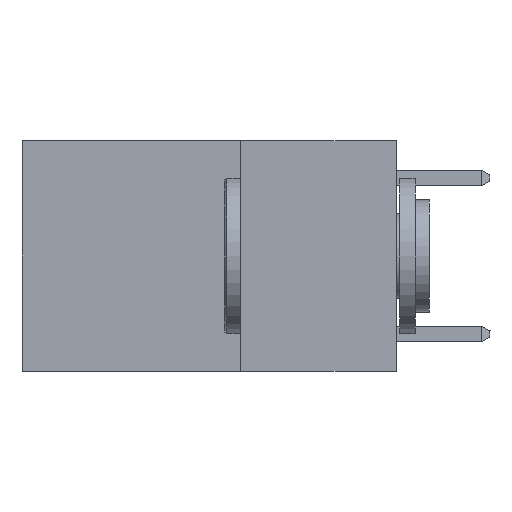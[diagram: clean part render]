
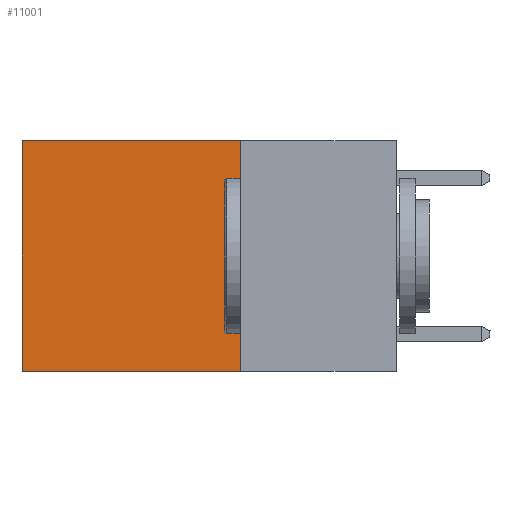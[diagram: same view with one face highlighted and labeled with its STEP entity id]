
A CAD part, left-side view. The second image highlights one B-rep face of the part: STEP entity #11001.
In plain terms, the highlighted planar face has unit normal (-1, 0, 0).
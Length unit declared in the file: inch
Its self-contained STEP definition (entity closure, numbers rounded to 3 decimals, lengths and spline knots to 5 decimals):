
#220 = PLANE ( 'NONE',  #23962 ) ;
#260 = CARTESIAN_POINT ( 'NONE',  ( 0.2625, 0.25, 0. ) ) ;
#681 = CARTESIAN_POINT ( 'NONE',  ( 0.2625, 0.25, -0.37 ) ) ;
#1607 = DIRECTION ( 'NONE',  ( 0., 0., -1. ) ) ;
#2259 = DIRECTION ( 'NONE',  ( 0., 1., 0. ) ) ;
#2545 = DIRECTION ( 'NONE',  ( 1., 0., 0. ) ) ;
#2746 = FACE_OUTER_BOUND ( 'NONE', #20581, .T. ) ;
#4446 = VECTOR ( 'NONE', #2259, 39.37008 ) ;
#4659 = ORIENTED_EDGE ( 'NONE', *, *, #26572, .T. ) ;
#5555 = ORIENTED_EDGE ( 'NONE', *, *, #27954, .F. ) ;
#5830 = LINE ( 'NONE', #10187, #11210 ) ;
#5943 = VERTEX_POINT ( 'NONE', #260 ) ;
#7524 = VERTEX_POINT ( 'NONE', #7734 ) ;
#7734 = CARTESIAN_POINT ( 'NONE',  ( 0.2625, 0.25, -0.37 ) ) ;
#8645 = VECTOR ( 'NONE', #18981, 39.37008 ) ;
#9068 = CARTESIAN_POINT ( 'NONE',  ( 0.2625, 0.25, 0. ) ) ;
#10187 = CARTESIAN_POINT ( 'NONE',  ( 0.2625, 0.25, 0. ) ) ;
#10566 = LINE ( 'NONE', #9068, #4446 ) ;
#11001 = ADVANCED_FACE ( 'NONE', ( #2746 ), #220, .F. ) ;
#11210 = VECTOR ( 'NONE', #16945, 39.37008 ) ;
#12831 = EDGE_CURVE ( 'NONE', #5943, #27323, #10566, .T. ) ;
#16250 = CARTESIAN_POINT ( 'NONE',  ( 0.2625, 0.25, 0. ) ) ;
#16945 = DIRECTION ( 'NONE',  ( 0., 0., -1. ) ) ;
#18523 = DIRECTION ( 'NONE',  ( 0., 0., -1. ) ) ;
#18981 = DIRECTION ( 'NONE',  ( 0., 1., 0. ) ) ;
#19715 = ORIENTED_EDGE ( 'NONE', *, *, #23733, .F. ) ;
#20019 = VERTEX_POINT ( 'NONE', #20889 ) ;
#20581 = EDGE_LOOP ( 'NONE', ( #4659, #5555, #19715, #26248 ) ) ;
#20889 = CARTESIAN_POINT ( 'NONE',  ( 0.2625, 0.6, -0.37 ) ) ;
#23003 = LINE ( 'NONE', #29030, #28418 ) ;
#23123 = CARTESIAN_POINT ( 'NONE',  ( 0.2625, 0.6, 0. ) ) ;
#23733 = EDGE_CURVE ( 'NONE', #5943, #7524, #5830, .T. ) ;
#23962 = AXIS2_PLACEMENT_3D ( 'NONE', #16250, #2545, #18523 ) ;
#26248 = ORIENTED_EDGE ( 'NONE', *, *, #12831, .T. ) ;
#26572 = EDGE_CURVE ( 'NONE', #27323, #20019, #23003, .T. ) ;
#27323 = VERTEX_POINT ( 'NONE', #23123 ) ;
#27616 = LINE ( 'NONE', #681, #8645 ) ;
#27954 = EDGE_CURVE ( 'NONE', #7524, #20019, #27616, .T. ) ;
#28418 = VECTOR ( 'NONE', #1607, 39.37008 ) ;
#29030 = CARTESIAN_POINT ( 'NONE',  ( 0.2625, 0.6, 0. ) ) ;
